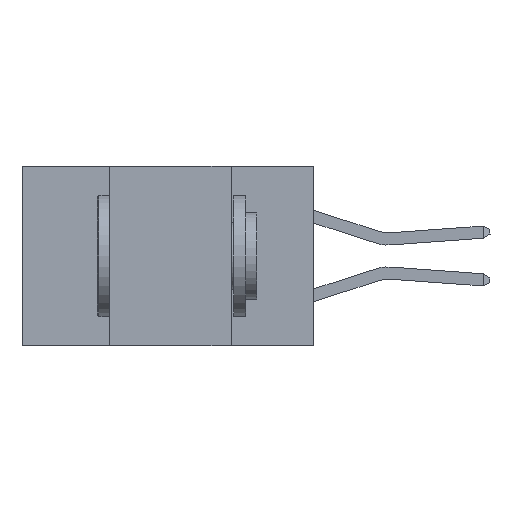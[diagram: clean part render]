
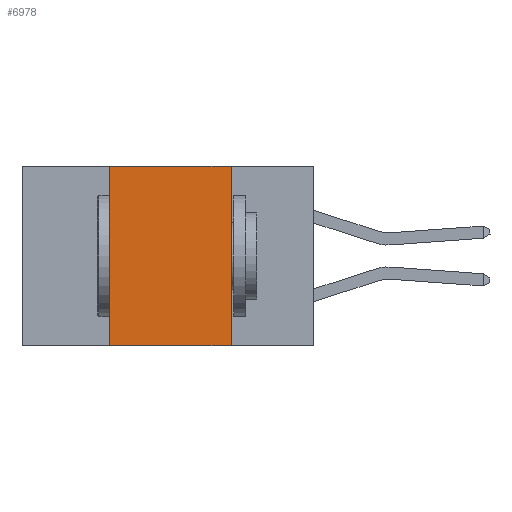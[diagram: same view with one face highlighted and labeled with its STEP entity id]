
A CAD part, left-side view. The second image highlights one B-rep face of the part: STEP entity #6978.
In plain terms, the highlighted planar face has unit normal (-1, 0, 0).
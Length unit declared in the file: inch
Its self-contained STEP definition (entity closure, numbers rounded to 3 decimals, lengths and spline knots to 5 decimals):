
#728 = EDGE_LOOP ( 'NONE', ( #15224, #6965, #6836, #8608 ) ) ;
#743 = EDGE_CURVE ( 'NONE', #14031, #6979, #13255, .T. ) ;
#865 = VECTOR ( 'NONE', #8847, 39.37008 ) ;
#1639 = VECTOR ( 'NONE', #14772, 39.37008 ) ;
#1817 = VERTEX_POINT ( 'NONE', #10511 ) ;
#1985 = PLANE ( 'NONE',  #9816 ) ;
#2044 = DIRECTION ( 'NONE',  ( 0., 0., -1. ) ) ;
#2143 = CARTESIAN_POINT ( 'NONE',  ( 0., 0.42, -0.37 ) ) ;
#3989 = EDGE_CURVE ( 'NONE', #4594, #14031, #11883, .T. ) ;
#4593 = CARTESIAN_POINT ( 'NONE',  ( 0., 0.17, 0. ) ) ;
#4594 = VERTEX_POINT ( 'NONE', #2143 ) ;
#4959 = VECTOR ( 'NONE', #9394, 39.37008 ) ;
#5189 = VECTOR ( 'NONE', #14562, 39.37008 ) ;
#5497 = EDGE_CURVE ( 'NONE', #4594, #1817, #10515, .T. ) ;
#5722 = CARTESIAN_POINT ( 'NONE',  ( 0., 0.17, 0. ) ) ;
#6555 = EDGE_CURVE ( 'NONE', #6979, #1817, #8711, .T. ) ;
#6836 = ORIENTED_EDGE ( 'NONE', *, *, #3989, .F. ) ;
#6965 = ORIENTED_EDGE ( 'NONE', *, *, #743, .F. ) ;
#6978 = ADVANCED_FACE ( 'NONE', ( #12777 ), #1985, .F. ) ;
#6979 = VERTEX_POINT ( 'NONE', #4593 ) ;
#8608 = ORIENTED_EDGE ( 'NONE', *, *, #5497, .T. ) ;
#8711 = LINE ( 'NONE', #5722, #4959 ) ;
#8847 = DIRECTION ( 'NONE',  ( 0., 0., 1. ) ) ;
#9394 = DIRECTION ( 'NONE',  ( 0., 0., -1. ) ) ;
#9816 = AXIS2_PLACEMENT_3D ( 'NONE', #14458, #15670, #2044 ) ;
#10511 = CARTESIAN_POINT ( 'NONE',  ( 0., 0.17, -0.37 ) ) ;
#10515 = LINE ( 'NONE', #12038, #5189 ) ;
#11883 = LINE ( 'NONE', #13759, #865 ) ;
#12038 = CARTESIAN_POINT ( 'NONE',  ( 0., 0.6, -0.37 ) ) ;
#12777 = FACE_OUTER_BOUND ( 'NONE', #728, .T. ) ;
#13255 = LINE ( 'NONE', #15652, #1639 ) ;
#13496 = CARTESIAN_POINT ( 'NONE',  ( 0., 0.42, 0. ) ) ;
#13759 = CARTESIAN_POINT ( 'NONE',  ( 0., 0.42, 0. ) ) ;
#14031 = VERTEX_POINT ( 'NONE', #13496 ) ;
#14458 = CARTESIAN_POINT ( 'NONE',  ( 0., 0.6, 0. ) ) ;
#14562 = DIRECTION ( 'NONE',  ( 0., -1., 0. ) ) ;
#14772 = DIRECTION ( 'NONE',  ( 0., -1., 0. ) ) ;
#15224 = ORIENTED_EDGE ( 'NONE', *, *, #6555, .F. ) ;
#15652 = CARTESIAN_POINT ( 'NONE',  ( 0., 0.6, 0. ) ) ;
#15670 = DIRECTION ( 'NONE',  ( 1., 0., 0. ) ) ;
